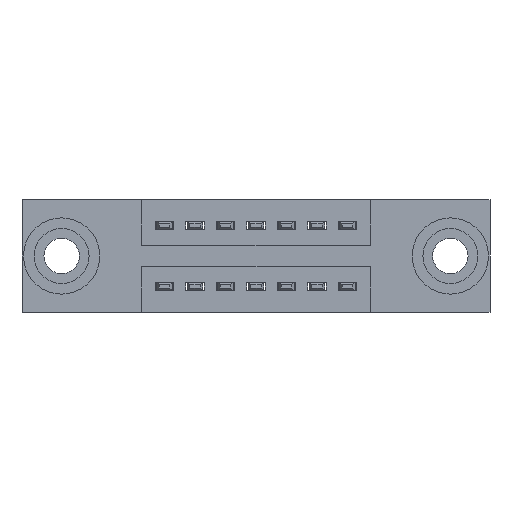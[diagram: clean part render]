
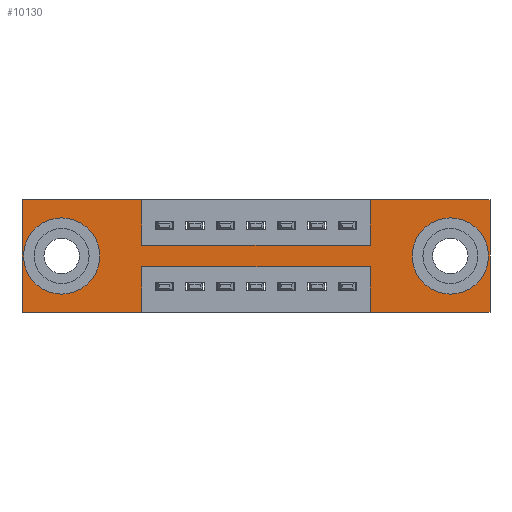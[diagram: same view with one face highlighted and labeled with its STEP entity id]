
A CAD part, front view. The second image highlights one B-rep face of the part: STEP entity #10130.
In plain terms, the highlighted planar face has unit normal (0, -1, 0).
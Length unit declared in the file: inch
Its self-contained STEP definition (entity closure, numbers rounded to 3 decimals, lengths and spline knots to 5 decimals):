
#86 = CARTESIAN_POINT ( 'NONE',  ( 0.3925, 0., -0.15 ) ) ;
#151 = VERTEX_POINT ( 'NONE', #6790 ) ;
#184 = EDGE_LOOP ( 'NONE', ( #8711, #7796 ) ) ;
#381 = CARTESIAN_POINT ( 'NONE',  ( 0., 0., 0. ) ) ;
#766 = EDGE_LOOP ( 'NONE', ( #806, #7226 ) ) ;
#800 = LINE ( 'NONE', #10306, #9722 ) ;
#806 = ORIENTED_EDGE ( 'NONE', *, *, #4638, .T. ) ;
#1013 = CARTESIAN_POINT ( 'NONE',  ( 1.1425, 0., -0.37 ) ) ;
#1101 = VERTEX_POINT ( 'NONE', #4847 ) ;
#1290 = DIRECTION ( 'NONE',  ( 0., 0., -1. ) ) ;
#1323 = VECTOR ( 'NONE', #1290, 39.37008 ) ;
#1395 = CARTESIAN_POINT ( 'NONE',  ( 0.3925, 0., 0. ) ) ;
#1398 = LINE ( 'NONE', #4652, #8236 ) ;
#1599 = AXIS2_PLACEMENT_3D ( 'NONE', #7808, #7696, #2808 ) ;
#1645 = CIRCLE ( 'NONE', #5164, 0.078 ) ;
#1646 = VERTEX_POINT ( 'NONE', #2970 ) ;
#1662 = DIRECTION ( 'NONE',  ( 0., 0., -1. ) ) ;
#1752 = DIRECTION ( 'NONE',  ( 1., 0., 0. ) ) ;
#1863 = DIRECTION ( 'NONE',  ( 0., 0., 1. ) ) ;
#1870 = EDGE_CURVE ( 'NONE', #1646, #6634, #4656, .T. ) ;
#1960 = VERTEX_POINT ( 'NONE', #3554 ) ;
#2010 = DIRECTION ( 'NONE',  ( 0., 1., 0. ) ) ;
#2146 = EDGE_CURVE ( 'NONE', #4469, #3075, #8023, .T. ) ;
#2226 = ORIENTED_EDGE ( 'NONE', *, *, #7601, .F. ) ;
#2238 = VECTOR ( 'NONE', #7041, 39.37008 ) ;
#2294 = FACE_BOUND ( 'NONE', #184, .T. ) ;
#2373 = ORIENTED_EDGE ( 'NONE', *, *, #7037, .F. ) ;
#2484 = CARTESIAN_POINT ( 'NONE',  ( 0.13, 0., -0.263 ) ) ;
#2586 = ORIENTED_EDGE ( 'NONE', *, *, #2146, .F. ) ;
#2617 = CARTESIAN_POINT ( 'NONE',  ( 0.3925, 0., -0.22 ) ) ;
#2673 = EDGE_LOOP ( 'NONE', ( #2373, #7780, #8229, #2226, #4459, #7434, #2586, #4766, #4784, #6005, #3136, #9617 ) ) ;
#2808 = DIRECTION ( 'NONE',  ( 0., 0., 1. ) ) ;
#2825 = VERTEX_POINT ( 'NONE', #8318 ) ;
#2877 = DIRECTION ( 'NONE',  ( 0., 0., -1. ) ) ;
#2889 = DIRECTION ( 'NONE',  ( 1., 0., 0. ) ) ;
#2970 = CARTESIAN_POINT ( 'NONE',  ( 0., 0., -0.37 ) ) ;
#3008 = CARTESIAN_POINT ( 'NONE',  ( 0.13, 0., -0.185 ) ) ;
#3046 = CARTESIAN_POINT ( 'NONE',  ( 0.13, 0., -0.107 ) ) ;
#3075 = VERTEX_POINT ( 'NONE', #3077 ) ;
#3077 = CARTESIAN_POINT ( 'NONE',  ( 1.1425, 0., 0. ) ) ;
#3080 = LINE ( 'NONE', #86, #8991 ) ;
#3136 = ORIENTED_EDGE ( 'NONE', *, *, #1870, .F. ) ;
#3459 = EDGE_CURVE ( 'NONE', #9388, #1646, #4259, .T. ) ;
#3554 = CARTESIAN_POINT ( 'NONE',  ( 1.405, 0., -0.107 ) ) ;
#3581 = DIRECTION ( 'NONE',  ( -1., 0., 0. ) ) ;
#3655 = LINE ( 'NONE', #1013, #5296 ) ;
#3721 = FACE_OUTER_BOUND ( 'NONE', #2673, .T. ) ;
#3779 = CARTESIAN_POINT ( 'NONE',  ( 1.1425, 0., -0.37 ) ) ;
#3799 = VECTOR ( 'NONE', #7731, 39.37008 ) ;
#3885 = CARTESIAN_POINT ( 'NONE',  ( 0.3925, 0., -0.37 ) ) ;
#3993 = EDGE_CURVE ( 'NONE', #5128, #4469, #3080, .T. ) ;
#4045 = VECTOR ( 'NONE', #6804, 39.37008 ) ;
#4259 = LINE ( 'NONE', #4882, #7862 ) ;
#4296 = DIRECTION ( 'NONE',  ( 0., 0., 1. ) ) ;
#4297 = LINE ( 'NONE', #381, #4779 ) ;
#4420 = EDGE_CURVE ( 'NONE', #2825, #1960, #1645, .T. ) ;
#4459 = ORIENTED_EDGE ( 'NONE', *, *, #6471, .F. ) ;
#4469 = VERTEX_POINT ( 'NONE', #5949 ) ;
#4638 = EDGE_CURVE ( 'NONE', #1960, #2825, #9271, .T. ) ;
#4652 = CARTESIAN_POINT ( 'NONE',  ( 0., 0., 0. ) ) ;
#4656 = LINE ( 'NONE', #7934, #2238 ) ;
#4766 = ORIENTED_EDGE ( 'NONE', *, *, #3993, .F. ) ;
#4779 = VECTOR ( 'NONE', #2889, 39.37008 ) ;
#4784 = ORIENTED_EDGE ( 'NONE', *, *, #6963, .F. ) ;
#4847 = CARTESIAN_POINT ( 'NONE',  ( 1.535, 0., -0.37 ) ) ;
#4881 = EDGE_CURVE ( 'NONE', #5540, #151, #5209, .T. ) ;
#4882 = CARTESIAN_POINT ( 'NONE',  ( 0., 0., -0.37 ) ) ;
#5128 = VERTEX_POINT ( 'NONE', #5378 ) ;
#5164 = AXIS2_PLACEMENT_3D ( 'NONE', #5258, #2010, #10115 ) ;
#5209 = LINE ( 'NONE', #2617, #4045 ) ;
#5258 = CARTESIAN_POINT ( 'NONE',  ( 1.405, 0., -0.185 ) ) ;
#5296 = VECTOR ( 'NONE', #4296, 39.37008 ) ;
#5378 = CARTESIAN_POINT ( 'NONE',  ( 0.3925, 0., -0.15 ) ) ;
#5497 = CIRCLE ( 'NONE', #7568, 0.078 ) ;
#5540 = VERTEX_POINT ( 'NONE', #8662 ) ;
#5605 = VERTEX_POINT ( 'NONE', #3046 ) ;
#5695 = LINE ( 'NONE', #1395, #1323 ) ;
#5720 = AXIS2_PLACEMENT_3D ( 'NONE', #8845, #6444, #9640 ) ;
#5831 = CARTESIAN_POINT ( 'NONE',  ( 1.535, 0., 0. ) ) ;
#5949 = CARTESIAN_POINT ( 'NONE',  ( 1.1425, 0., -0.15 ) ) ;
#6005 = ORIENTED_EDGE ( 'NONE', *, *, #7238, .F. ) ;
#6013 = VECTOR ( 'NONE', #3581, 39.37008 ) ;
#6253 = CARTESIAN_POINT ( 'NONE',  ( 1.535, 0., 0. ) ) ;
#6282 = DIRECTION ( 'NONE',  ( 0., 0., 1. ) ) ;
#6444 = DIRECTION ( 'NONE',  ( 0., 1., 0. ) ) ;
#6471 = EDGE_CURVE ( 'NONE', #10578, #1101, #6495, .T. ) ;
#6495 = LINE ( 'NONE', #6253, #3799 ) ;
#6592 = CARTESIAN_POINT ( 'NONE',  ( 0., 0., 0. ) ) ;
#6634 = VERTEX_POINT ( 'NONE', #6592 ) ;
#6671 = DIRECTION ( 'NONE',  ( 0., -1., 0. ) ) ;
#6790 = CARTESIAN_POINT ( 'NONE',  ( 0.3925, 0., -0.22 ) ) ;
#6795 = CARTESIAN_POINT ( 'NONE',  ( 1.1425, 0., 0. ) ) ;
#6804 = DIRECTION ( 'NONE',  ( -1., 0., 0. ) ) ;
#6963 = EDGE_CURVE ( 'NONE', #9134, #5128, #5695, .T. ) ;
#7034 = EDGE_CURVE ( 'NONE', #10682, #5605, #9339, .T. ) ;
#7037 = EDGE_CURVE ( 'NONE', #151, #9388, #800, .T. ) ;
#7041 = DIRECTION ( 'NONE',  ( 0., 0., 1. ) ) ;
#7074 = DIRECTION ( 'NONE',  ( 0., 1., 0. ) ) ;
#7226 = ORIENTED_EDGE ( 'NONE', *, *, #4420, .T. ) ;
#7238 = EDGE_CURVE ( 'NONE', #6634, #9134, #4297, .T. ) ;
#7382 = CARTESIAN_POINT ( 'NONE',  ( 0., 0., -0.37 ) ) ;
#7428 = DIRECTION ( 'NONE',  ( 1., 0., 0. ) ) ;
#7434 = ORIENTED_EDGE ( 'NONE', *, *, #9453, .F. ) ;
#7565 = EDGE_CURVE ( 'NONE', #9223, #5540, #3655, .T. ) ;
#7568 = AXIS2_PLACEMENT_3D ( 'NONE', #3008, #7074, #6282 ) ;
#7601 = EDGE_CURVE ( 'NONE', #1101, #9223, #9764, .T. ) ;
#7696 = DIRECTION ( 'NONE',  ( 0., 1., 0. ) ) ;
#7731 = DIRECTION ( 'NONE',  ( 0., 0., -1. ) ) ;
#7780 = ORIENTED_EDGE ( 'NONE', *, *, #4881, .F. ) ;
#7796 = ORIENTED_EDGE ( 'NONE', *, *, #7034, .T. ) ;
#7808 = CARTESIAN_POINT ( 'NONE',  ( 0.13, 0., -0.185 ) ) ;
#7862 = VECTOR ( 'NONE', #8212, 39.37008 ) ;
#7934 = CARTESIAN_POINT ( 'NONE',  ( 0., 0., 0. ) ) ;
#8023 = LINE ( 'NONE', #6795, #8428 ) ;
#8212 = DIRECTION ( 'NONE',  ( -1., 0., 0. ) ) ;
#8229 = ORIENTED_EDGE ( 'NONE', *, *, #7565, .F. ) ;
#8236 = VECTOR ( 'NONE', #7428, 39.37008 ) ;
#8318 = CARTESIAN_POINT ( 'NONE',  ( 1.405, 0., -0.263 ) ) ;
#8367 = FACE_BOUND ( 'NONE', #766, .T. ) ;
#8428 = VECTOR ( 'NONE', #1863, 39.37008 ) ;
#8662 = CARTESIAN_POINT ( 'NONE',  ( 1.1425, 0., -0.22 ) ) ;
#8711 = ORIENTED_EDGE ( 'NONE', *, *, #9935, .T. ) ;
#8845 = CARTESIAN_POINT ( 'NONE',  ( 1.405, 0., -0.185 ) ) ;
#8991 = VECTOR ( 'NONE', #1752, 39.37008 ) ;
#8992 = PLANE ( 'NONE',  #10397 ) ;
#9069 = CARTESIAN_POINT ( 'NONE',  ( 0., 0., -0.37 ) ) ;
#9134 = VERTEX_POINT ( 'NONE', #9974 ) ;
#9223 = VERTEX_POINT ( 'NONE', #3779 ) ;
#9271 = CIRCLE ( 'NONE', #5720, 0.078 ) ;
#9339 = CIRCLE ( 'NONE', #1599, 0.078 ) ;
#9388 = VERTEX_POINT ( 'NONE', #3885 ) ;
#9453 = EDGE_CURVE ( 'NONE', #3075, #10578, #1398, .T. ) ;
#9617 = ORIENTED_EDGE ( 'NONE', *, *, #3459, .F. ) ;
#9640 = DIRECTION ( 'NONE',  ( 0., 0., -1. ) ) ;
#9722 = VECTOR ( 'NONE', #2877, 39.37008 ) ;
#9764 = LINE ( 'NONE', #9069, #6013 ) ;
#9935 = EDGE_CURVE ( 'NONE', #5605, #10682, #5497, .T. ) ;
#9974 = CARTESIAN_POINT ( 'NONE',  ( 0.3925, 0., 0. ) ) ;
#10115 = DIRECTION ( 'NONE',  ( 0., 0., -1. ) ) ;
#10130 = ADVANCED_FACE ( 'NONE', ( #8367, #2294, #3721 ), #8992, .T. ) ;
#10306 = CARTESIAN_POINT ( 'NONE',  ( 0.3925, 0., -0.37 ) ) ;
#10397 = AXIS2_PLACEMENT_3D ( 'NONE', #7382, #6671, #1662 ) ;
#10578 = VERTEX_POINT ( 'NONE', #5831 ) ;
#10682 = VERTEX_POINT ( 'NONE', #2484 ) ;
